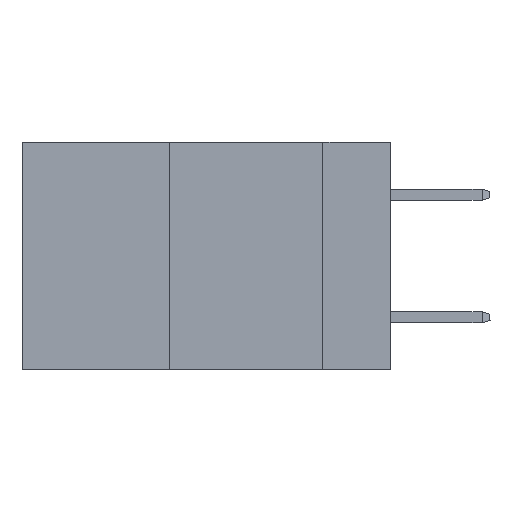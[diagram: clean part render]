
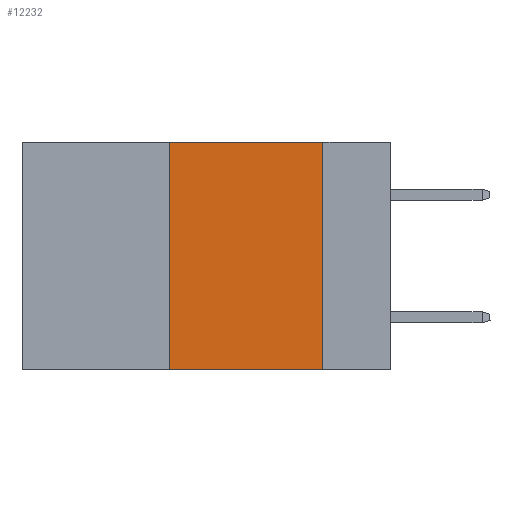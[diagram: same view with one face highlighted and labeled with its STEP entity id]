
A CAD part, left-side view. The second image highlights one B-rep face of the part: STEP entity #12232.
In plain terms, the highlighted planar face has unit normal (-1, 0, 0).
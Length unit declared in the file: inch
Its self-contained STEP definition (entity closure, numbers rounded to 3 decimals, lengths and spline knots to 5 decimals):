
#367 = VECTOR ( 'NONE', #964, 39.37008 ) ;
#417 = DIRECTION ( 'NONE',  ( 0., -1., 0. ) ) ;
#964 = DIRECTION ( 'NONE',  ( 0., -1., 0. ) ) ;
#2521 = EDGE_LOOP ( 'NONE', ( #19643, #9786, #16835, #17154 ) ) ;
#2531 = CARTESIAN_POINT ( 'NONE',  ( 0., 0.11, 0. ) ) ;
#4840 = LINE ( 'NONE', #7941, #6959 ) ;
#5348 = DIRECTION ( 'NONE',  ( 0., 0., -1. ) ) ;
#6071 = CARTESIAN_POINT ( 'NONE',  ( 0., 0.6, 0. ) ) ;
#6335 = DIRECTION ( 'NONE',  ( 0., 0., 1. ) ) ;
#6959 = VECTOR ( 'NONE', #6335, 39.37008 ) ;
#7146 = CARTESIAN_POINT ( 'NONE',  ( 0., 0.36, 0. ) ) ;
#7262 = VECTOR ( 'NONE', #417, 39.37008 ) ;
#7419 = DIRECTION ( 'NONE',  ( 0., 0., -1. ) ) ;
#7425 = LINE ( 'NONE', #17007, #367 ) ;
#7640 = EDGE_CURVE ( 'NONE', #15591, #10573, #7425, .T. ) ;
#7941 = CARTESIAN_POINT ( 'NONE',  ( 0., 0.36, 0. ) ) ;
#8113 = EDGE_CURVE ( 'NONE', #14276, #14271, #8782, .T. ) ;
#8782 = LINE ( 'NONE', #15122, #7262 ) ;
#8795 = PLANE ( 'NONE',  #10713 ) ;
#9094 = EDGE_CURVE ( 'NONE', #15591, #14276, #4840, .T. ) ;
#9786 = ORIENTED_EDGE ( 'NONE', *, *, #8113, .F. ) ;
#10573 = VERTEX_POINT ( 'NONE', #19544 ) ;
#10713 = AXIS2_PLACEMENT_3D ( 'NONE', #6071, #15356, #7419 ) ;
#11703 = CARTESIAN_POINT ( 'NONE',  ( 0., 0.11, 0. ) ) ;
#11924 = LINE ( 'NONE', #11703, #13085 ) ;
#12232 = ADVANCED_FACE ( 'NONE', ( #17592 ), #8795, .F. ) ;
#13085 = VECTOR ( 'NONE', #5348, 39.37008 ) ;
#14271 = VERTEX_POINT ( 'NONE', #2531 ) ;
#14276 = VERTEX_POINT ( 'NONE', #7146 ) ;
#15122 = CARTESIAN_POINT ( 'NONE',  ( 0., 0.6, 0. ) ) ;
#15356 = DIRECTION ( 'NONE',  ( 1., 0., 0. ) ) ;
#15591 = VERTEX_POINT ( 'NONE', #20206 ) ;
#16835 = ORIENTED_EDGE ( 'NONE', *, *, #9094, .F. ) ;
#17007 = CARTESIAN_POINT ( 'NONE',  ( 0., 0.6, -0.37 ) ) ;
#17154 = ORIENTED_EDGE ( 'NONE', *, *, #7640, .T. ) ;
#17592 = FACE_OUTER_BOUND ( 'NONE', #2521, .T. ) ;
#19544 = CARTESIAN_POINT ( 'NONE',  ( 0., 0.11, -0.37 ) ) ;
#19643 = ORIENTED_EDGE ( 'NONE', *, *, #20018, .F. ) ;
#20018 = EDGE_CURVE ( 'NONE', #14271, #10573, #11924, .T. ) ;
#20206 = CARTESIAN_POINT ( 'NONE',  ( 0., 0.36, -0.37 ) ) ;
